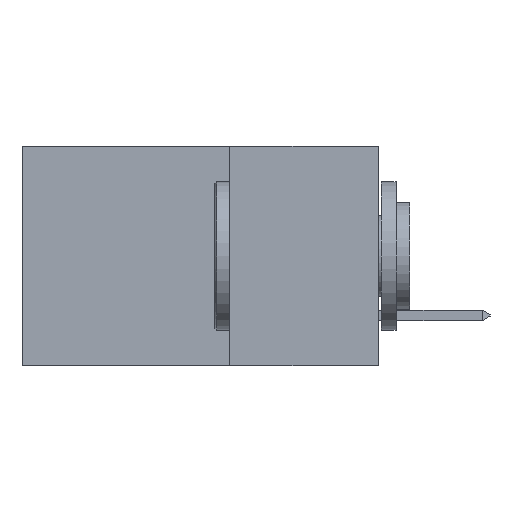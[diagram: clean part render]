
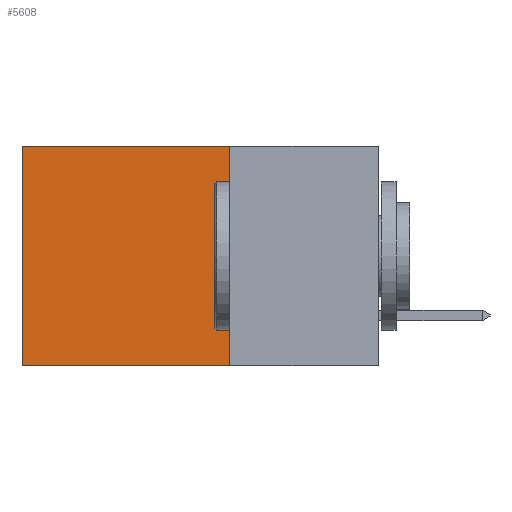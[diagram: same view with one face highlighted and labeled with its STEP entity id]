
A CAD part, left-side view. The second image highlights one B-rep face of the part: STEP entity #5608.
In plain terms, the highlighted planar face has unit normal (-1, 0, 0).
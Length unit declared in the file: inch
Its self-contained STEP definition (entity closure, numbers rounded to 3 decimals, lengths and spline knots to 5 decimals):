
#5 = VERTEX_POINT ( 'NONE', #5122 ) ;
#209 = CARTESIAN_POINT ( 'NONE',  ( 0.298, 0.25, 0. ) ) ;
#309 = AXIS2_PLACEMENT_3D ( 'NONE', #8392, #8861, #8850 ) ;
#331 = CARTESIAN_POINT ( 'NONE',  ( 0.298, 0.6, 0. ) ) ;
#2220 = CARTESIAN_POINT ( 'NONE',  ( 0.298, 0.25, -0.37 ) ) ;
#2561 = LINE ( 'NONE', #209, #10397 ) ;
#2580 = ORIENTED_EDGE ( 'NONE', *, *, #2787, .F. ) ;
#2588 = CARTESIAN_POINT ( 'NONE',  ( 0.298, 0.25, 0. ) ) ;
#2625 = DIRECTION ( 'NONE',  ( 0., 1., 0. ) ) ;
#2650 = FACE_OUTER_BOUND ( 'NONE', #5381, .T. ) ;
#2668 = EDGE_CURVE ( 'NONE', #6175, #5, #8488, .T. ) ;
#2787 = EDGE_CURVE ( 'NONE', #8499, #7309, #7523, .T. ) ;
#2884 = VECTOR ( 'NONE', #2625, 39.37008 ) ;
#3157 = LINE ( 'NONE', #2220, #2884 ) ;
#3176 = VECTOR ( 'NONE', #6892, 39.37008 ) ;
#3745 = DIRECTION ( 'NONE',  ( 0., 0., -1. ) ) ;
#3985 = ORIENTED_EDGE ( 'NONE', *, *, #5990, .F. ) ;
#4083 = DIRECTION ( 'NONE',  ( 0., 1., 0. ) ) ;
#4112 = EDGE_CURVE ( 'NONE', #8499, #6175, #2561, .T. ) ;
#4140 = ORIENTED_EDGE ( 'NONE', *, *, #4112, .T. ) ;
#4201 = VECTOR ( 'NONE', #3745, 39.37008 ) ;
#5122 = CARTESIAN_POINT ( 'NONE',  ( 0.298, 0.6, -0.37 ) ) ;
#5260 = CARTESIAN_POINT ( 'NONE',  ( 0.298, 0.6, 0. ) ) ;
#5381 = EDGE_LOOP ( 'NONE', ( #6024, #3985, #2580, #4140 ) ) ;
#5608 = ADVANCED_FACE ( 'NONE', ( #2650 ), #9445, .F. ) ;
#5990 = EDGE_CURVE ( 'NONE', #7309, #5, #3157, .T. ) ;
#6024 = ORIENTED_EDGE ( 'NONE', *, *, #2668, .T. ) ;
#6175 = VERTEX_POINT ( 'NONE', #331 ) ;
#6892 = DIRECTION ( 'NONE',  ( 0., 0., -1. ) ) ;
#7309 = VERTEX_POINT ( 'NONE', #9898 ) ;
#7523 = LINE ( 'NONE', #10261, #3176 ) ;
#8392 = CARTESIAN_POINT ( 'NONE',  ( 0.298, 0.25, 0. ) ) ;
#8488 = LINE ( 'NONE', #5260, #4201 ) ;
#8499 = VERTEX_POINT ( 'NONE', #2588 ) ;
#8850 = DIRECTION ( 'NONE',  ( 0., 0., -1. ) ) ;
#8861 = DIRECTION ( 'NONE',  ( 1., 0., 0. ) ) ;
#9445 = PLANE ( 'NONE',  #309 ) ;
#9898 = CARTESIAN_POINT ( 'NONE',  ( 0.298, 0.25, -0.37 ) ) ;
#10261 = CARTESIAN_POINT ( 'NONE',  ( 0.298, 0.25, 0. ) ) ;
#10397 = VECTOR ( 'NONE', #4083, 39.37008 ) ;
